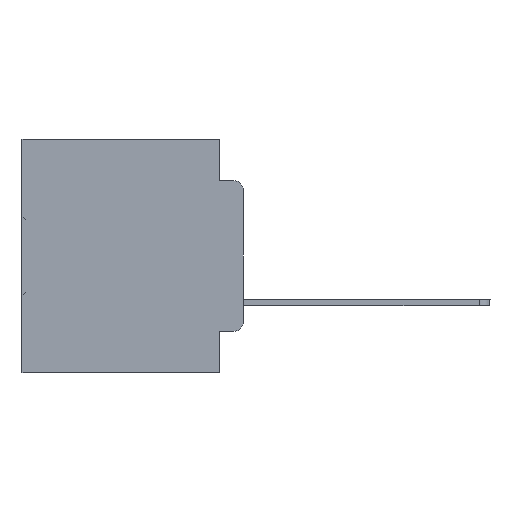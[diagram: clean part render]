
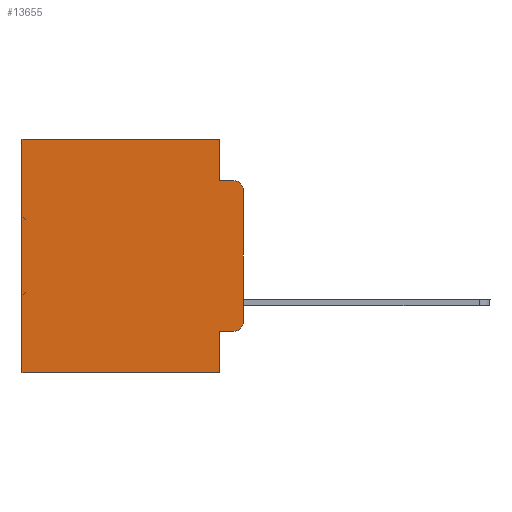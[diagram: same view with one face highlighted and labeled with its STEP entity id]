
A CAD part, left-side view. The second image highlights one B-rep face of the part: STEP entity #13655.
In plain terms, the highlighted planar face has unit normal (-1, 0, 0).
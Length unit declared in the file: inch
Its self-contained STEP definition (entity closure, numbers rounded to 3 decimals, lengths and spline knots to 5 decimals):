
#23 = VERTEX_POINT ( 'NONE', #2746 ) ;
#2237 = VERTEX_POINT ( 'NONE', #8890 ) ;
#2383 = DIRECTION ( 'NONE',  ( 0., -1., 0. ) ) ;
#2401 = FACE_OUTER_BOUND ( 'NONE', #32977, .T. ) ;
#2746 = CARTESIAN_POINT ( 'NONE',  ( 0.298, 0.02, -0.4115 ) ) ;
#3051 = CARTESIAN_POINT ( 'NONE',  ( 0.298, 0.02, -0.1085 ) ) ;
#4452 = LINE ( 'NONE', #18336, #35488 ) ;
#4681 = PLANE ( 'NONE',  #10419 ) ;
#5208 = LINE ( 'NONE', #16645, #15042 ) ;
#5753 = AXIS2_PLACEMENT_3D ( 'NONE', #31046, #22375, #33857 ) ;
#6309 = VECTOR ( 'NONE', #37091, 39.37008 ) ;
#6673 = LINE ( 'NONE', #23770, #9914 ) ;
#6887 = DIRECTION ( 'NONE',  ( 0., 0., -1. ) ) ;
#7247 = VERTEX_POINT ( 'NONE', #23713 ) ;
#7857 = DIRECTION ( 'NONE',  ( 1., 0., 0. ) ) ;
#8066 = EDGE_CURVE ( 'NONE', #2237, #21695, #14232, .T. ) ;
#8515 = VERTEX_POINT ( 'NONE', #11017 ) ;
#8753 = CIRCLE ( 'NONE', #5753, 0.02 ) ;
#8890 = CARTESIAN_POINT ( 'NONE',  ( 0.298, 0.051, 0. ) ) ;
#9017 = CARTESIAN_POINT ( 'NONE',  ( 0.298, 0., -0.3915 ) ) ;
#9914 = VECTOR ( 'NONE', #11075, 39.37008 ) ;
#10056 = EDGE_CURVE ( 'NONE', #8515, #23, #5208, .T. ) ;
#10419 = AXIS2_PLACEMENT_3D ( 'NONE', #25342, #7857, #19313 ) ;
#10779 = VECTOR ( 'NONE', #24406, 39.37008 ) ;
#10831 = ORIENTED_EDGE ( 'NONE', *, *, #25200, .T. ) ;
#11017 = CARTESIAN_POINT ( 'NONE',  ( 0.298, 0.051, -0.4115 ) ) ;
#11075 = DIRECTION ( 'NONE',  ( 0., 0., -1. ) ) ;
#11363 = ORIENTED_EDGE ( 'NONE', *, *, #37043, .T. ) ;
#12242 = ORIENTED_EDGE ( 'NONE', *, *, #34417, .F. ) ;
#12736 = LINE ( 'NONE', #24022, #10779 ) ;
#12771 = DIRECTION ( 'NONE',  ( 0., -1., 0. ) ) ;
#13655 = ADVANCED_FACE ( 'NONE', ( #2401 ), #4681, .F. ) ;
#14232 = LINE ( 'NONE', #25359, #32383 ) ;
#14656 = EDGE_CURVE ( 'NONE', #7247, #19869, #27904, .T. ) ;
#15042 = VECTOR ( 'NONE', #2383, 39.37008 ) ;
#16411 = VERTEX_POINT ( 'NONE', #9017 ) ;
#16645 = CARTESIAN_POINT ( 'NONE',  ( 0.298, 0.051, -0.4115 ) ) ;
#17497 = CARTESIAN_POINT ( 'NONE',  ( 0.298, 0.051, 0. ) ) ;
#17682 = LINE ( 'NONE', #17497, #6309 ) ;
#18336 = CARTESIAN_POINT ( 'NONE',  ( 0.298, 0.051, 0. ) ) ;
#18788 = VECTOR ( 'NONE', #36255, 39.37008 ) ;
#19238 = EDGE_CURVE ( 'NONE', #29708, #19869, #35350, .T. ) ;
#19313 = DIRECTION ( 'NONE',  ( 0., 0., -1. ) ) ;
#19406 = CARTESIAN_POINT ( 'NONE',  ( 0.298, 0.473, 0. ) ) ;
#19869 = VERTEX_POINT ( 'NONE', #25881 ) ;
#21138 = CARTESIAN_POINT ( 'NONE',  ( 0.298, 0.051, -0.5 ) ) ;
#21483 = VERTEX_POINT ( 'NONE', #29765 ) ;
#21695 = VERTEX_POINT ( 'NONE', #19406 ) ;
#22375 = DIRECTION ( 'NONE',  ( -1., 0., 0. ) ) ;
#22377 = ORIENTED_EDGE ( 'NONE', *, *, #19238, .F. ) ;
#22977 = DIRECTION ( 'NONE',  ( -1., 0., 0. ) ) ;
#23713 = CARTESIAN_POINT ( 'NONE',  ( 0.298, 0., -0.1085 ) ) ;
#23770 = CARTESIAN_POINT ( 'NONE',  ( 0.298, 0.473, 0. ) ) ;
#24022 = CARTESIAN_POINT ( 'NONE',  ( 0.298, 0., 0. ) ) ;
#24406 = DIRECTION ( 'NONE',  ( 0., 0., -1. ) ) ;
#24784 = LINE ( 'NONE', #27797, #18788 ) ;
#25200 = EDGE_CURVE ( 'NONE', #21695, #21483, #6673, .T. ) ;
#25342 = CARTESIAN_POINT ( 'NONE',  ( 0.298, 0., 0. ) ) ;
#25359 = CARTESIAN_POINT ( 'NONE',  ( 0.298, 0., 0. ) ) ;
#25881 = CARTESIAN_POINT ( 'NONE',  ( 0.298, 0.02, -0.0885 ) ) ;
#26669 = AXIS2_PLACEMENT_3D ( 'NONE', #3051, #22977, #36913 ) ;
#27797 = CARTESIAN_POINT ( 'NONE',  ( 0.298, 0., -0.5 ) ) ;
#27904 = CIRCLE ( 'NONE', #26669, 0.02 ) ;
#28099 = ORIENTED_EDGE ( 'NONE', *, *, #10056, .T. ) ;
#28592 = ORIENTED_EDGE ( 'NONE', *, *, #14656, .T. ) ;
#29516 = EDGE_CURVE ( 'NONE', #7247, #16411, #12736, .T. ) ;
#29708 = VERTEX_POINT ( 'NONE', #36628 ) ;
#29750 = ORIENTED_EDGE ( 'NONE', *, *, #36614, .F. ) ;
#29765 = CARTESIAN_POINT ( 'NONE',  ( 0.298, 0.473, -0.5 ) ) ;
#29938 = ORIENTED_EDGE ( 'NONE', *, *, #8066, .T. ) ;
#31046 = CARTESIAN_POINT ( 'NONE',  ( 0.298, 0.02, -0.3915 ) ) ;
#31191 = DIRECTION ( 'NONE',  ( 0., 1., 0. ) ) ;
#31233 = EDGE_CURVE ( 'NONE', #2237, #29708, #4452, .T. ) ;
#32383 = VECTOR ( 'NONE', #31191, 39.37008 ) ;
#32721 = CARTESIAN_POINT ( 'NONE',  ( 0.298, 0.051, -0.0885 ) ) ;
#32794 = ORIENTED_EDGE ( 'NONE', *, *, #31233, .F. ) ;
#32977 = EDGE_LOOP ( 'NONE', ( #37113, #28592, #22377, #32794, #29938, #10831, #12242, #29750, #28099, #11363 ) ) ;
#33650 = VECTOR ( 'NONE', #12771, 39.37008 ) ;
#33857 = DIRECTION ( 'NONE',  ( 0., 0., -1. ) ) ;
#34417 = EDGE_CURVE ( 'NONE', #34599, #21483, #24784, .T. ) ;
#34599 = VERTEX_POINT ( 'NONE', #21138 ) ;
#35350 = LINE ( 'NONE', #32721, #33650 ) ;
#35488 = VECTOR ( 'NONE', #6887, 39.37008 ) ;
#36255 = DIRECTION ( 'NONE',  ( 0., 1., 0. ) ) ;
#36614 = EDGE_CURVE ( 'NONE', #8515, #34599, #17682, .T. ) ;
#36628 = CARTESIAN_POINT ( 'NONE',  ( 0.298, 0.051, -0.0885 ) ) ;
#36913 = DIRECTION ( 'NONE',  ( 0., 0., -1. ) ) ;
#37043 = EDGE_CURVE ( 'NONE', #23, #16411, #8753, .T. ) ;
#37091 = DIRECTION ( 'NONE',  ( 0., 0., -1. ) ) ;
#37113 = ORIENTED_EDGE ( 'NONE', *, *, #29516, .F. ) ;
